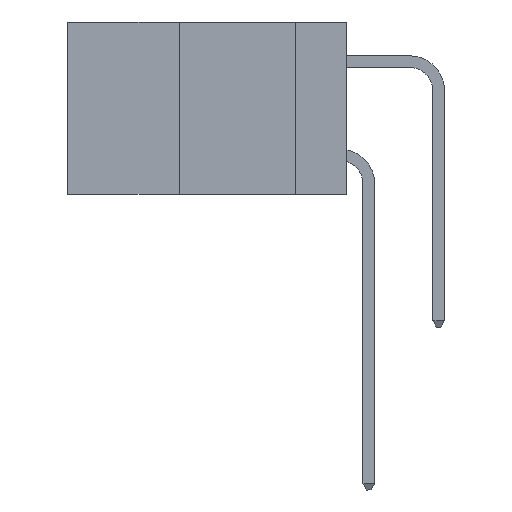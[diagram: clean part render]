
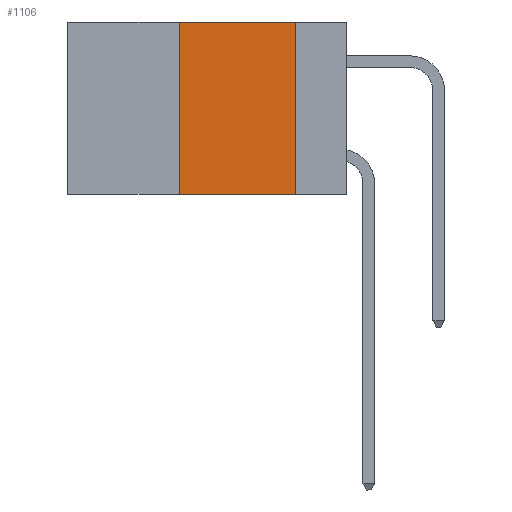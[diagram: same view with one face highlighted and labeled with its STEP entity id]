
A CAD part, left-side view. The second image highlights one B-rep face of the part: STEP entity #1106.
In plain terms, the highlighted planar face has unit normal (-1, 0, 0).
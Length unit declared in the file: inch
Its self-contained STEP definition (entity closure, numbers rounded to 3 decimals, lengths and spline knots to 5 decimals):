
#382 = ORIENTED_EDGE ( 'NONE', *, *, #7049, .F. ) ;
#1094 = CARTESIAN_POINT ( 'NONE',  ( 0., 0.11, 0. ) ) ;
#1106 = ADVANCED_FACE ( 'NONE', ( #5183 ), #17249, .F. ) ;
#1286 = DIRECTION ( 'NONE',  ( 0., 0., -1. ) ) ;
#1919 = VECTOR ( 'NONE', #15076, 39.37008 ) ;
#2246 = VERTEX_POINT ( 'NONE', #3293 ) ;
#3038 = CARTESIAN_POINT ( 'NONE',  ( 0., 0.6, 0. ) ) ;
#3203 = EDGE_CURVE ( 'NONE', #5472, #12385, #11522, .T. ) ;
#3293 = CARTESIAN_POINT ( 'NONE',  ( 0., 0.36, 0. ) ) ;
#3465 = ORIENTED_EDGE ( 'NONE', *, *, #3203, .T. ) ;
#3681 = ORIENTED_EDGE ( 'NONE', *, *, #11875, .F. ) ;
#4318 = CARTESIAN_POINT ( 'NONE',  ( 0., 0.6, -0.37 ) ) ;
#4736 = EDGE_LOOP ( 'NONE', ( #3681, #19459, #382, #3465 ) ) ;
#5183 = FACE_OUTER_BOUND ( 'NONE', #4736, .T. ) ;
#5210 = DIRECTION ( 'NONE',  ( 1., 0., 0. ) ) ;
#5472 = VERTEX_POINT ( 'NONE', #11367 ) ;
#5481 = DIRECTION ( 'NONE',  ( 0., -1., 0. ) ) ;
#6199 = CARTESIAN_POINT ( 'NONE',  ( 0., 0.36, 0. ) ) ;
#6843 = VECTOR ( 'NONE', #5481, 39.37008 ) ;
#7049 = EDGE_CURVE ( 'NONE', #5472, #2246, #18547, .T. ) ;
#8011 = DIRECTION ( 'NONE',  ( 0., 0., 1. ) ) ;
#9505 = VECTOR ( 'NONE', #8011, 39.37008 ) ;
#10507 = AXIS2_PLACEMENT_3D ( 'NONE', #3038, #5210, #1286 ) ;
#11367 = CARTESIAN_POINT ( 'NONE',  ( 0., 0.36, -0.37 ) ) ;
#11522 = LINE ( 'NONE', #4318, #1919 ) ;
#11526 = LINE ( 'NONE', #17588, #6843 ) ;
#11875 = EDGE_CURVE ( 'NONE', #18470, #12385, #16768, .T. ) ;
#12249 = CARTESIAN_POINT ( 'NONE',  ( 0., 0.11, 0. ) ) ;
#12385 = VERTEX_POINT ( 'NONE', #13148 ) ;
#13148 = CARTESIAN_POINT ( 'NONE',  ( 0., 0.11, -0.37 ) ) ;
#15076 = DIRECTION ( 'NONE',  ( 0., -1., 0. ) ) ;
#16768 = LINE ( 'NONE', #1094, #20630 ) ;
#17249 = PLANE ( 'NONE',  #10507 ) ;
#17588 = CARTESIAN_POINT ( 'NONE',  ( 0., 0.6, 0. ) ) ;
#18470 = VERTEX_POINT ( 'NONE', #12249 ) ;
#18547 = LINE ( 'NONE', #6199, #9505 ) ;
#18624 = DIRECTION ( 'NONE',  ( 0., 0., -1. ) ) ;
#19459 = ORIENTED_EDGE ( 'NONE', *, *, #22320, .F. ) ;
#20630 = VECTOR ( 'NONE', #18624, 39.37008 ) ;
#22320 = EDGE_CURVE ( 'NONE', #2246, #18470, #11526, .T. ) ;
